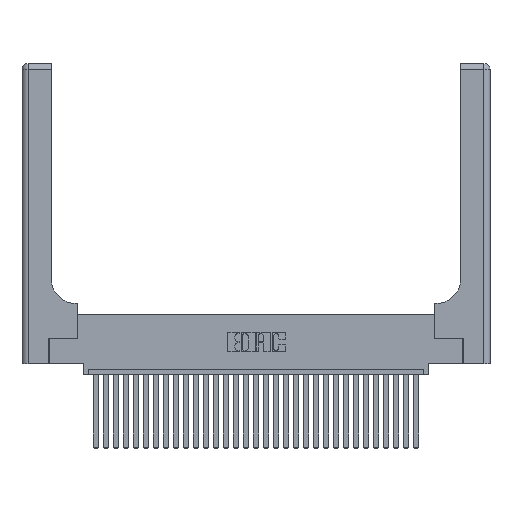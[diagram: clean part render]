
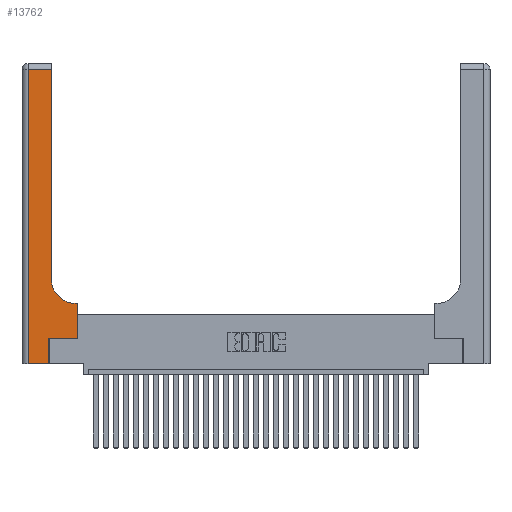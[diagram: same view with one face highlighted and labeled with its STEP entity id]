
A CAD part, top view. The second image highlights one B-rep face of the part: STEP entity #13762.
In plain terms, the highlighted planar face has unit normal (0, 0, 1).
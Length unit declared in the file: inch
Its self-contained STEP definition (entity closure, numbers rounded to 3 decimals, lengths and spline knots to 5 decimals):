
#372 = VECTOR ( 'NONE', #24663, 39.37008 ) ;
#1004 = ORIENTED_EDGE ( 'NONE', *, *, #9566, .T. ) ;
#1353 = VERTEX_POINT ( 'NONE', #4650 ) ;
#2461 = CARTESIAN_POINT ( 'NONE',  ( 0.269, 0., 0.37 ) ) ;
#2520 = EDGE_CURVE ( 'NONE', #30986, #30895, #15917, .T. ) ;
#2763 = ORIENTED_EDGE ( 'NONE', *, *, #15890, .T. ) ;
#2982 = ORIENTED_EDGE ( 'NONE', *, *, #30759, .T. ) ;
#3515 = VERTEX_POINT ( 'NONE', #18318 ) ;
#3521 = LINE ( 'NONE', #14814, #20456 ) ;
#4299 = CARTESIAN_POINT ( 'NONE',  ( 0.2915, 2.94, 0.37 ) ) ;
#4503 = LINE ( 'NONE', #13557, #21789 ) ;
#4650 = CARTESIAN_POINT ( 'NONE',  ( 0.06, 2.94, 0.37 ) ) ;
#4678 = ORIENTED_EDGE ( 'NONE', *, *, #5004, .T. ) ;
#4711 = DIRECTION ( 'NONE',  ( -1., 0., 0. ) ) ;
#4839 = VECTOR ( 'NONE', #4711, 39.37008 ) ;
#4990 = CARTESIAN_POINT ( 'NONE',  ( 0.2915, 0.6, 0.37 ) ) ;
#5004 = EDGE_CURVE ( 'NONE', #1353, #11350, #4503, .T. ) ;
#5362 = ORIENTED_EDGE ( 'NONE', *, *, #23995, .T. ) ;
#5385 = LINE ( 'NONE', #8404, #23887 ) ;
#5506 = ORIENTED_EDGE ( 'NONE', *, *, #29468, .T. ) ;
#6283 = DIRECTION ( 'NONE',  ( 0., 0., -1. ) ) ;
#6457 = DIRECTION ( 'NONE',  ( 1., 0., 0. ) ) ;
#6672 = CARTESIAN_POINT ( 'NONE',  ( 0.269, 0., 0.37 ) ) ;
#7571 = LINE ( 'NONE', #6672, #372 ) ;
#8404 = CARTESIAN_POINT ( 'NONE',  ( 0.2915, 3., 0.37 ) ) ;
#9566 = EDGE_CURVE ( 'NONE', #15599, #27535, #7571, .T. ) ;
#10344 = CARTESIAN_POINT ( 'NONE',  ( 0.5585, 0.25, 0.37 ) ) ;
#10442 = FACE_OUTER_BOUND ( 'NONE', #28929, .T. ) ;
#10577 = CARTESIAN_POINT ( 'NONE',  ( 0.5415, 0.85, 0.37 ) ) ;
#11215 = LINE ( 'NONE', #4990, #4839 ) ;
#11350 = VERTEX_POINT ( 'NONE', #23653 ) ;
#12394 = ORIENTED_EDGE ( 'NONE', *, *, #27319, .T. ) ;
#12395 = DIRECTION ( 'NONE',  ( 1., 0., 0. ) ) ;
#13010 = DIRECTION ( 'NONE',  ( 0., 0., -1. ) ) ;
#13037 = DIRECTION ( 'NONE',  ( 0., 1., 0. ) ) ;
#13557 = CARTESIAN_POINT ( 'NONE',  ( 0.06, 3., 0.37 ) ) ;
#13762 = ADVANCED_FACE ( 'NONE', ( #10442 ), #22406, .F. ) ;
#13988 = CARTESIAN_POINT ( 'NONE',  ( 0.5585, 0.6, 0.37 ) ) ;
#14814 = CARTESIAN_POINT ( 'NONE',  ( 0., 2.94, 0.37 ) ) ;
#15599 = VERTEX_POINT ( 'NONE', #2461 ) ;
#15890 = EDGE_CURVE ( 'NONE', #30895, #16881, #5385, .T. ) ;
#15917 = CIRCLE ( 'NONE', #30820, 0.25 ) ;
#16881 = VERTEX_POINT ( 'NONE', #4299 ) ;
#18318 = CARTESIAN_POINT ( 'NONE',  ( 0.5585, 0.25, 0.37 ) ) ;
#18405 = DIRECTION ( 'NONE',  ( 0., -1., 0. ) ) ;
#18668 = CARTESIAN_POINT ( 'NONE',  ( 0., 0., 0.37 ) ) ;
#19130 = VECTOR ( 'NONE', #26807, 39.37008 ) ;
#19864 = LINE ( 'NONE', #10344, #19130 ) ;
#20098 = AXIS2_PLACEMENT_3D ( 'NONE', #29875, #6283, #20490 ) ;
#20456 = VECTOR ( 'NONE', #29382, 39.37008 ) ;
#20490 = DIRECTION ( 'NONE',  ( -1., 0., 0. ) ) ;
#21789 = VECTOR ( 'NONE', #18405, 39.37008 ) ;
#21887 = VERTEX_POINT ( 'NONE', #13988 ) ;
#21959 = CARTESIAN_POINT ( 'NONE',  ( 0.269, 0.25, 0.37 ) ) ;
#22406 = PLANE ( 'NONE',  #20098 ) ;
#22859 = CARTESIAN_POINT ( 'NONE',  ( 0.5415, 0.6, 0.37 ) ) ;
#23321 = CARTESIAN_POINT ( 'NONE',  ( 0.269, 0.25, 0.37 ) ) ;
#23381 = VECTOR ( 'NONE', #12395, 39.37008 ) ;
#23653 = CARTESIAN_POINT ( 'NONE',  ( 0.06, 0., 0.37 ) ) ;
#23887 = VECTOR ( 'NONE', #13037, 39.37008 ) ;
#23995 = EDGE_CURVE ( 'NONE', #27535, #3515, #30126, .T. ) ;
#24663 = DIRECTION ( 'NONE',  ( 0., 1., 0. ) ) ;
#25165 = CARTESIAN_POINT ( 'NONE',  ( 0.2915, 0.85, 0.37 ) ) ;
#26807 = DIRECTION ( 'NONE',  ( 0., 1., 0. ) ) ;
#27175 = EDGE_CURVE ( 'NONE', #21887, #30986, #11215, .T. ) ;
#27319 = EDGE_CURVE ( 'NONE', #3515, #21887, #19864, .T. ) ;
#27535 = VERTEX_POINT ( 'NONE', #23321 ) ;
#28817 = VECTOR ( 'NONE', #6457, 39.37008 ) ;
#28832 = ORIENTED_EDGE ( 'NONE', *, *, #2520, .T. ) ;
#28929 = EDGE_LOOP ( 'NONE', ( #2763, #2982, #4678, #5506, #1004, #5362, #12394, #30400, #28832 ) ) ;
#29382 = DIRECTION ( 'NONE',  ( -1., 0., 0. ) ) ;
#29468 = EDGE_CURVE ( 'NONE', #11350, #15599, #29565, .T. ) ;
#29565 = LINE ( 'NONE', #18668, #28817 ) ;
#29772 = DIRECTION ( 'NONE',  ( 1., 0., 0. ) ) ;
#29875 = CARTESIAN_POINT ( 'NONE',  ( 0., 3., 0.37 ) ) ;
#30126 = LINE ( 'NONE', #21959, #23381 ) ;
#30400 = ORIENTED_EDGE ( 'NONE', *, *, #27175, .T. ) ;
#30759 = EDGE_CURVE ( 'NONE', #16881, #1353, #3521, .T. ) ;
#30820 = AXIS2_PLACEMENT_3D ( 'NONE', #10577, #13010, #29772 ) ;
#30895 = VERTEX_POINT ( 'NONE', #25165 ) ;
#30986 = VERTEX_POINT ( 'NONE', #22859 ) ;
